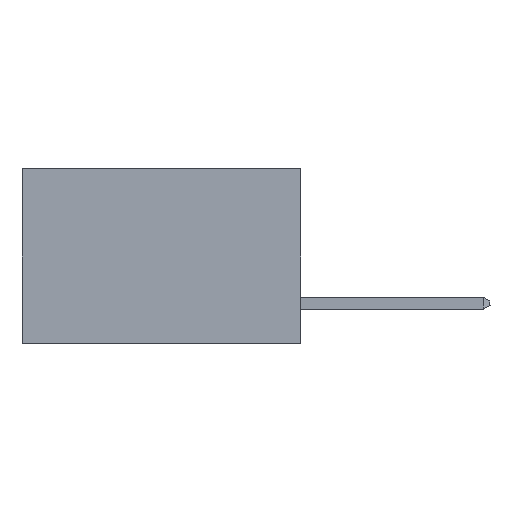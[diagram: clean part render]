
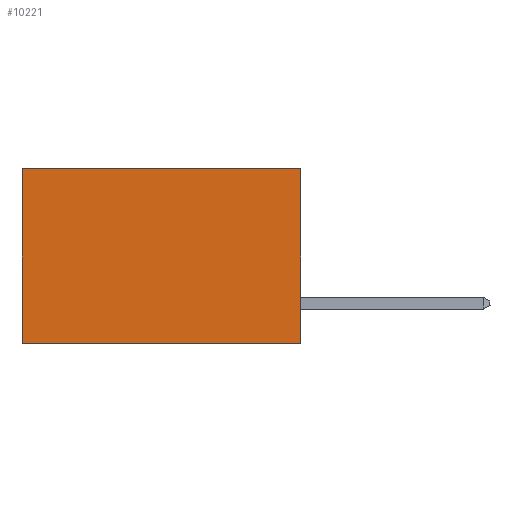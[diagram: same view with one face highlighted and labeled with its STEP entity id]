
A CAD part, left-side view. The second image highlights one B-rep face of the part: STEP entity #10221.
In plain terms, the highlighted planar face has unit normal (-1, 0, 0).
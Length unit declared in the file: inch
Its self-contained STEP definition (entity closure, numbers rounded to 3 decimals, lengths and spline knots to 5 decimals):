
#79 = CARTESIAN_POINT ( 'NONE',  ( 0.277, 0.59, -0.37 ) ) ;
#121 = EDGE_CURVE ( 'NONE', #11951, #1092, #15470, .T. ) ;
#354 = DIRECTION ( 'NONE',  ( 0., 1., 0. ) ) ;
#575 = CARTESIAN_POINT ( 'NONE',  ( 0.277, 0., 0. ) ) ;
#729 = VECTOR ( 'NONE', #354, 39.37008 ) ;
#1012 = LINE ( 'NONE', #7021, #5092 ) ;
#1092 = VERTEX_POINT ( 'NONE', #7444 ) ;
#2780 = VECTOR ( 'NONE', #17804, 39.37008 ) ;
#2928 = EDGE_CURVE ( 'NONE', #6930, #6631, #10438, .T. ) ;
#3140 = ORIENTED_EDGE ( 'NONE', *, *, #11158, .F. ) ;
#3373 = PLANE ( 'NONE',  #7236 ) ;
#3914 = DIRECTION ( 'NONE',  ( 0., 1., 0. ) ) ;
#4860 = ORIENTED_EDGE ( 'NONE', *, *, #7769, .T. ) ;
#4949 = CARTESIAN_POINT ( 'NONE',  ( 0.277, 0., -0.37 ) ) ;
#5092 = VECTOR ( 'NONE', #3914, 39.37008 ) ;
#5319 = LINE ( 'NONE', #575, #729 ) ;
#6527 = DIRECTION ( 'NONE',  ( 1., 0., 0. ) ) ;
#6631 = VERTEX_POINT ( 'NONE', #14603 ) ;
#6930 = VERTEX_POINT ( 'NONE', #10468 ) ;
#7021 = CARTESIAN_POINT ( 'NONE',  ( 0.277, 0., -0.37 ) ) ;
#7139 = DIRECTION ( 'NONE',  ( 0., 0., -1. ) ) ;
#7236 = AXIS2_PLACEMENT_3D ( 'NONE', #4949, #6527, #16996 ) ;
#7444 = CARTESIAN_POINT ( 'NONE',  ( 0.277, 0.59, -0.37 ) ) ;
#7769 = EDGE_CURVE ( 'NONE', #6930, #11951, #5319, .T. ) ;
#9059 = CARTESIAN_POINT ( 'NONE',  ( 0.277, 0.59, 0. ) ) ;
#9364 = ORIENTED_EDGE ( 'NONE', *, *, #2928, .F. ) ;
#10221 = ADVANCED_FACE ( 'NONE', ( #10449 ), #3373, .F. ) ;
#10428 = EDGE_LOOP ( 'NONE', ( #14248, #3140, #9364, #4860 ) ) ;
#10438 = LINE ( 'NONE', #17338, #2780 ) ;
#10449 = FACE_OUTER_BOUND ( 'NONE', #10428, .T. ) ;
#10468 = CARTESIAN_POINT ( 'NONE',  ( 0.277, 0., 0. ) ) ;
#11158 = EDGE_CURVE ( 'NONE', #6631, #1092, #1012, .T. ) ;
#11951 = VERTEX_POINT ( 'NONE', #9059 ) ;
#14248 = ORIENTED_EDGE ( 'NONE', *, *, #121, .T. ) ;
#14603 = CARTESIAN_POINT ( 'NONE',  ( 0.277, 0., -0.37 ) ) ;
#15470 = LINE ( 'NONE', #79, #18971 ) ;
#16996 = DIRECTION ( 'NONE',  ( 0., 0., -1. ) ) ;
#17338 = CARTESIAN_POINT ( 'NONE',  ( 0.277, 0., -0.37 ) ) ;
#17804 = DIRECTION ( 'NONE',  ( 0., 0., -1. ) ) ;
#18971 = VECTOR ( 'NONE', #7139, 39.37008 ) ;
